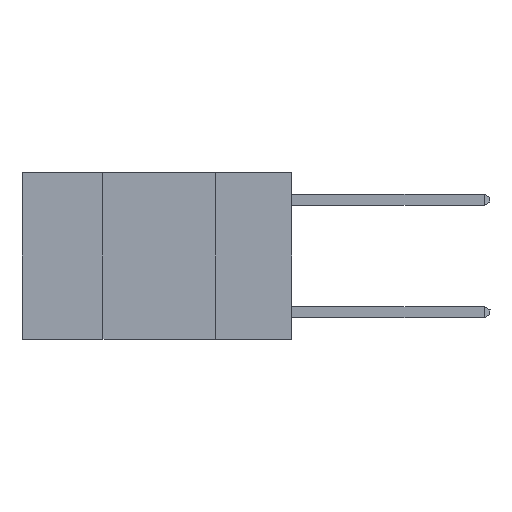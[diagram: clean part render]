
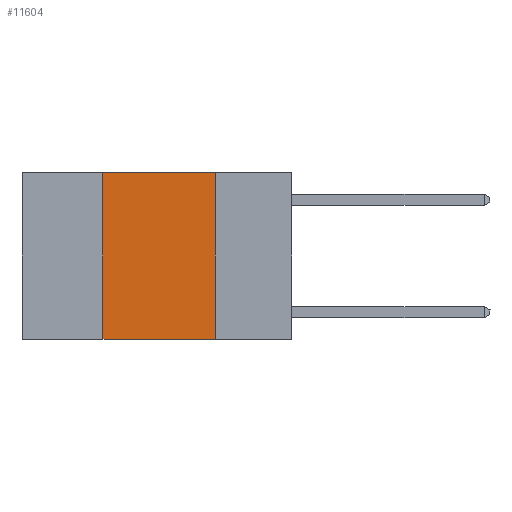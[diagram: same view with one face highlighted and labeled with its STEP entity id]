
A CAD part, left-side view. The second image highlights one B-rep face of the part: STEP entity #11604.
In plain terms, the highlighted planar face has unit normal (-1, 0, 0).
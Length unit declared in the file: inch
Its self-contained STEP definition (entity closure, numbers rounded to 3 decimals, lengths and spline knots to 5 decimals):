
#276 = ORIENTED_EDGE ( 'NONE', *, *, #1778, .F. ) ;
#282 = AXIS2_PLACEMENT_3D ( 'NONE', #7137, #502, #8184 ) ;
#502 = DIRECTION ( 'NONE',  ( 1., 0., 0. ) ) ;
#822 = CARTESIAN_POINT ( 'NONE',  ( 0., 0.42, -0.37 ) ) ;
#830 = CARTESIAN_POINT ( 'NONE',  ( 0., 0.17, 0. ) ) ;
#945 = EDGE_CURVE ( 'NONE', #13426, #1856, #13527, .T. ) ;
#1101 = FACE_OUTER_BOUND ( 'NONE', #7742, .T. ) ;
#1778 = EDGE_CURVE ( 'NONE', #8381, #12614, #13505, .T. ) ;
#1856 = VERTEX_POINT ( 'NONE', #10047 ) ;
#2244 = EDGE_CURVE ( 'NONE', #13426, #8381, #3651, .T. ) ;
#2286 = EDGE_CURVE ( 'NONE', #12614, #1856, #7751, .T. ) ;
#2452 = VECTOR ( 'NONE', #6437, 39.37008 ) ;
#2876 = DIRECTION ( 'NONE',  ( 0., -1., 0. ) ) ;
#3064 = ORIENTED_EDGE ( 'NONE', *, *, #945, .T. ) ;
#3078 = DIRECTION ( 'NONE',  ( 0., 0., 1. ) ) ;
#3188 = CARTESIAN_POINT ( 'NONE',  ( 0., 0.6, 0. ) ) ;
#3651 = LINE ( 'NONE', #6050, #11351 ) ;
#5167 = VECTOR ( 'NONE', #7190, 39.37008 ) ;
#6050 = CARTESIAN_POINT ( 'NONE',  ( 0., 0.42, 0. ) ) ;
#6437 = DIRECTION ( 'NONE',  ( 0., -1., 0. ) ) ;
#7137 = CARTESIAN_POINT ( 'NONE',  ( 0., 0.6, 0. ) ) ;
#7190 = DIRECTION ( 'NONE',  ( 0., 0., -1. ) ) ;
#7742 = EDGE_LOOP ( 'NONE', ( #8615, #276, #11931, #3064 ) ) ;
#7751 = LINE ( 'NONE', #830, #5167 ) ;
#8029 = CARTESIAN_POINT ( 'NONE',  ( 0., 0.6, -0.37 ) ) ;
#8184 = DIRECTION ( 'NONE',  ( 0., 0., -1. ) ) ;
#8363 = CARTESIAN_POINT ( 'NONE',  ( 0., 0.42, 0. ) ) ;
#8381 = VERTEX_POINT ( 'NONE', #8363 ) ;
#8600 = VECTOR ( 'NONE', #2876, 39.37008 ) ;
#8615 = ORIENTED_EDGE ( 'NONE', *, *, #2286, .F. ) ;
#10047 = CARTESIAN_POINT ( 'NONE',  ( 0., 0.17, -0.37 ) ) ;
#10147 = PLANE ( 'NONE',  #282 ) ;
#10430 = CARTESIAN_POINT ( 'NONE',  ( 0., 0.17, 0. ) ) ;
#11351 = VECTOR ( 'NONE', #3078, 39.37008 ) ;
#11604 = ADVANCED_FACE ( 'NONE', ( #1101 ), #10147, .F. ) ;
#11931 = ORIENTED_EDGE ( 'NONE', *, *, #2244, .F. ) ;
#12614 = VERTEX_POINT ( 'NONE', #10430 ) ;
#13426 = VERTEX_POINT ( 'NONE', #822 ) ;
#13505 = LINE ( 'NONE', #3188, #2452 ) ;
#13527 = LINE ( 'NONE', #8029, #8600 ) ;
